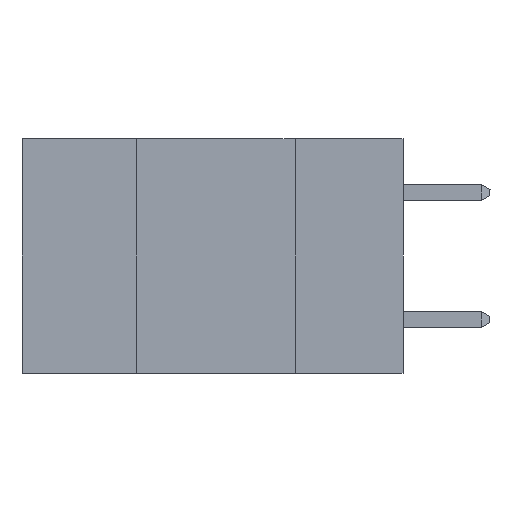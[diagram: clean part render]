
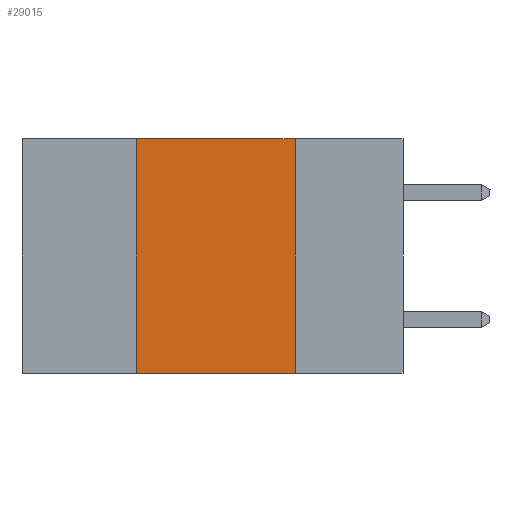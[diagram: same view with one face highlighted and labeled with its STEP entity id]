
A CAD part, left-side view. The second image highlights one B-rep face of the part: STEP entity #29015.
In plain terms, the highlighted planar face has unit normal (-1, 0, 0).
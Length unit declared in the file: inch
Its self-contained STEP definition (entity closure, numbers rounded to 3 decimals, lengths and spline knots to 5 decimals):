
#940 = ORIENTED_EDGE ( 'NONE', *, *, #20010, .F. ) ;
#1792 = VECTOR ( 'NONE', #18479, 39.37008 ) ;
#3136 = LINE ( 'NONE', #26072, #21239 ) ;
#3747 = VERTEX_POINT ( 'NONE', #4332 ) ;
#4332 = CARTESIAN_POINT ( 'NONE',  ( 0., 0.42, -0.37 ) ) ;
#6130 = VERTEX_POINT ( 'NONE', #16683 ) ;
#6424 = VECTOR ( 'NONE', #19878, 39.37008 ) ;
#7191 = CARTESIAN_POINT ( 'NONE',  ( 0., 0.17, -0.37 ) ) ;
#9247 = CARTESIAN_POINT ( 'NONE',  ( 0., 0.42, 0. ) ) ;
#10230 = ORIENTED_EDGE ( 'NONE', *, *, #28709, .T. ) ;
#10652 = DIRECTION ( 'NONE',  ( 1., 0., 0. ) ) ;
#11372 = EDGE_CURVE ( 'NONE', #6130, #20948, #12760, .T. ) ;
#12760 = LINE ( 'NONE', #26774, #6424 ) ;
#13424 = DIRECTION ( 'NONE',  ( 0., -1., 0. ) ) ;
#14420 = DIRECTION ( 'NONE',  ( 0., -1., 0. ) ) ;
#15015 = ORIENTED_EDGE ( 'NONE', *, *, #25888, .F. ) ;
#16683 = CARTESIAN_POINT ( 'NONE',  ( 0., 0.17, 0. ) ) ;
#18031 = LINE ( 'NONE', #29774, #28245 ) ;
#18479 = DIRECTION ( 'NONE',  ( 0., 0., 1. ) ) ;
#19878 = DIRECTION ( 'NONE',  ( 0., 0., -1. ) ) ;
#20010 = EDGE_CURVE ( 'NONE', #27333, #6130, #18031, .T. ) ;
#20948 = VERTEX_POINT ( 'NONE', #7191 ) ;
#21239 = VECTOR ( 'NONE', #14420, 39.37008 ) ;
#22277 = AXIS2_PLACEMENT_3D ( 'NONE', #24685, #10652, #26995 ) ;
#22375 = PLANE ( 'NONE',  #22277 ) ;
#22677 = FACE_OUTER_BOUND ( 'NONE', #25085, .T. ) ;
#23097 = CARTESIAN_POINT ( 'NONE',  ( 0., 0.42, 0. ) ) ;
#24685 = CARTESIAN_POINT ( 'NONE',  ( 0., 0.6, 0. ) ) ;
#25085 = EDGE_LOOP ( 'NONE', ( #28511, #940, #15015, #10230 ) ) ;
#25888 = EDGE_CURVE ( 'NONE', #3747, #27333, #27525, .T. ) ;
#26072 = CARTESIAN_POINT ( 'NONE',  ( 0., 0.6, -0.37 ) ) ;
#26774 = CARTESIAN_POINT ( 'NONE',  ( 0., 0.17, 0. ) ) ;
#26995 = DIRECTION ( 'NONE',  ( 0., 0., -1. ) ) ;
#27333 = VERTEX_POINT ( 'NONE', #9247 ) ;
#27525 = LINE ( 'NONE', #23097, #1792 ) ;
#28245 = VECTOR ( 'NONE', #13424, 39.37008 ) ;
#28511 = ORIENTED_EDGE ( 'NONE', *, *, #11372, .F. ) ;
#28709 = EDGE_CURVE ( 'NONE', #3747, #20948, #3136, .T. ) ;
#29015 = ADVANCED_FACE ( 'NONE', ( #22677 ), #22375, .F. ) ;
#29774 = CARTESIAN_POINT ( 'NONE',  ( 0., 0.6, 0. ) ) ;
